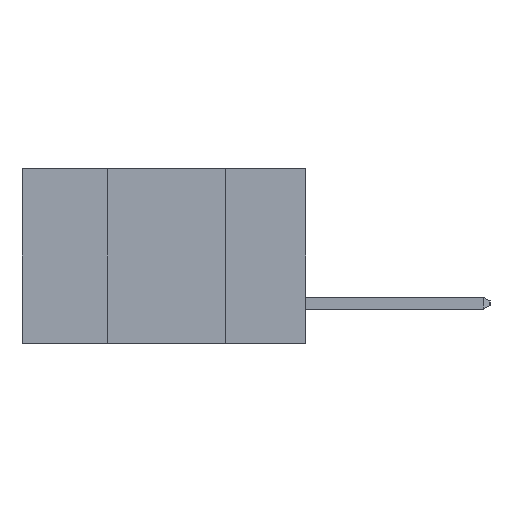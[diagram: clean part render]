
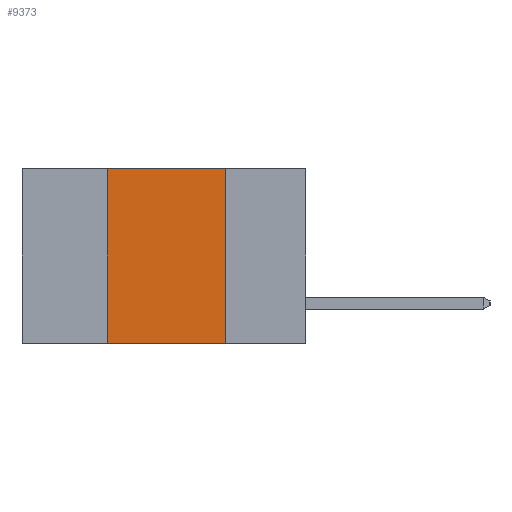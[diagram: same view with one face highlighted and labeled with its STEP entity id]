
A CAD part, left-side view. The second image highlights one B-rep face of the part: STEP entity #9373.
In plain terms, the highlighted planar face has unit normal (-1, 0, 0).
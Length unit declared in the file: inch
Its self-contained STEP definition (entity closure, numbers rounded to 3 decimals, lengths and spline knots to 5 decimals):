
#427 = LINE ( 'NONE', #10771, #5636 ) ;
#470 = EDGE_LOOP ( 'NONE', ( #4454, #4429, #4399, #4369 ) ) ;
#940 = DIRECTION ( 'NONE',  ( 0., 0., 1. ) ) ;
#1026 = VECTOR ( 'NONE', #1985, 39.37008 ) ;
#1568 = DIRECTION ( 'NONE',  ( 0., 0., -1. ) ) ;
#1726 = EDGE_CURVE ( 'NONE', #7351, #10779, #427, .T. ) ;
#1985 = DIRECTION ( 'NONE',  ( 0., -1., 0. ) ) ;
#2996 = CARTESIAN_POINT ( 'NONE',  ( 0., 0.42, 0. ) ) ;
#3849 = LINE ( 'NONE', #7077, #1026 ) ;
#3873 = CARTESIAN_POINT ( 'NONE',  ( 0., 0.17, -0.37 ) ) ;
#3881 = LINE ( 'NONE', #4072, #11663 ) ;
#4072 = CARTESIAN_POINT ( 'NONE',  ( 0., 0.42, -0.37 ) ) ;
#4369 = ORIENTED_EDGE ( 'NONE', *, *, #10914, .T. ) ;
#4399 = ORIENTED_EDGE ( 'NONE', *, *, #9632, .F. ) ;
#4429 = ORIENTED_EDGE ( 'NONE', *, *, #9001, .F. ) ;
#4454 = ORIENTED_EDGE ( 'NONE', *, *, #1726, .F. ) ;
#5636 = VECTOR ( 'NONE', #10505, 39.37008 ) ;
#5668 = PLANE ( 'NONE',  #11212 ) ;
#6673 = CARTESIAN_POINT ( 'NONE',  ( 0., 0.6, 0. ) ) ;
#7077 = CARTESIAN_POINT ( 'NONE',  ( 0., 0.6, -0.37 ) ) ;
#7351 = VERTEX_POINT ( 'NONE', #9945 ) ;
#7674 = DIRECTION ( 'NONE',  ( 1., 0., 0. ) ) ;
#7970 = FACE_OUTER_BOUND ( 'NONE', #470, .T. ) ;
#8799 = CARTESIAN_POINT ( 'NONE',  ( 0., 0.6, 0. ) ) ;
#8827 = VERTEX_POINT ( 'NONE', #11384 ) ;
#9001 = EDGE_CURVE ( 'NONE', #10886, #7351, #12092, .T. ) ;
#9373 = ADVANCED_FACE ( 'NONE', ( #7970 ), #5668, .F. ) ;
#9632 = EDGE_CURVE ( 'NONE', #8827, #10886, #3881, .T. ) ;
#9945 = CARTESIAN_POINT ( 'NONE',  ( 0., 0.17, 0. ) ) ;
#10505 = DIRECTION ( 'NONE',  ( 0., 0., -1. ) ) ;
#10771 = CARTESIAN_POINT ( 'NONE',  ( 0., 0.17, -0.37 ) ) ;
#10779 = VERTEX_POINT ( 'NONE', #3873 ) ;
#10886 = VERTEX_POINT ( 'NONE', #2996 ) ;
#10914 = EDGE_CURVE ( 'NONE', #8827, #10779, #3849, .T. ) ;
#11212 = AXIS2_PLACEMENT_3D ( 'NONE', #6673, #7674, #1568 ) ;
#11384 = CARTESIAN_POINT ( 'NONE',  ( 0., 0.42, -0.37 ) ) ;
#11663 = VECTOR ( 'NONE', #940, 39.37008 ) ;
#11808 = VECTOR ( 'NONE', #12531, 39.37008 ) ;
#12092 = LINE ( 'NONE', #8799, #11808 ) ;
#12531 = DIRECTION ( 'NONE',  ( 0., -1., 0. ) ) ;
